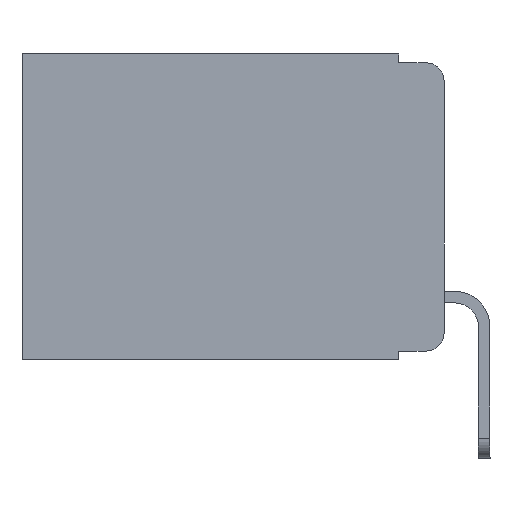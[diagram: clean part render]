
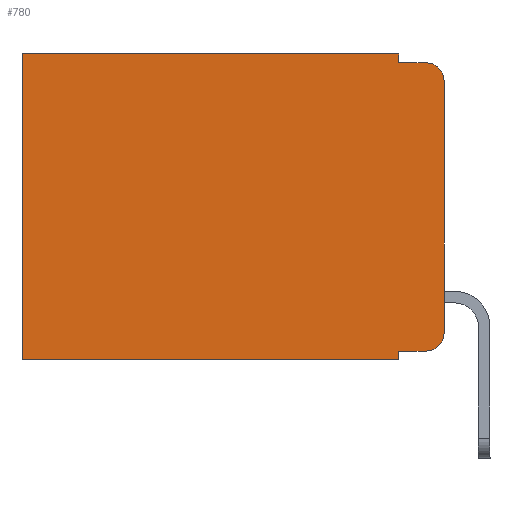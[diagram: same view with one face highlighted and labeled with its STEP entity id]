
A CAD part, left-side view. The second image highlights one B-rep face of the part: STEP entity #780.
In plain terms, the highlighted planar face has unit normal (-1, 0, 0).
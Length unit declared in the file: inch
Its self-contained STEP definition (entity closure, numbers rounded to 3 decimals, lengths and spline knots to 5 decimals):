
#149 = EDGE_CURVE ( 'NONE', #5123, #1282, #10667, .T. ) ;
#304 = EDGE_CURVE ( 'NONE', #12042, #5918, #4848, .T. ) ;
#460 = DIRECTION ( 'NONE',  ( 0., -1., 0. ) ) ;
#780 = ADVANCED_FACE ( 'NONE', ( #3816 ), #7426, .F. ) ;
#827 = CARTESIAN_POINT ( 'NONE',  ( 0.298, 0., -0.343 ) ) ;
#1242 = CARTESIAN_POINT ( 'NONE',  ( 0.298, 0.02, -0.03 ) ) ;
#1282 = VERTEX_POINT ( 'NONE', #5396 ) ;
#1289 = DIRECTION ( 'NONE',  ( 0., 0., -1. ) ) ;
#1403 = CARTESIAN_POINT ( 'NONE',  ( 0.298, 0.051, -0.01 ) ) ;
#1415 = CIRCLE ( 'NONE', #5154, 0.02 ) ;
#1849 = DIRECTION ( 'NONE',  ( 0., 1., 0. ) ) ;
#2070 = EDGE_CURVE ( 'NONE', #13044, #11261, #13061, .T. ) ;
#2125 = CARTESIAN_POINT ( 'NONE',  ( 0.298, 0.051, -0.333 ) ) ;
#2136 = VECTOR ( 'NONE', #10372, 39.37008 ) ;
#2192 = DIRECTION ( 'NONE',  ( 1., 0., 0. ) ) ;
#2296 = VECTOR ( 'NONE', #3104, 39.37008 ) ;
#2339 = CARTESIAN_POINT ( 'NONE',  ( 0.298, 0.051, -0.01 ) ) ;
#2659 = VECTOR ( 'NONE', #7117, 39.37008 ) ;
#2788 = LINE ( 'NONE', #7250, #11934 ) ;
#2936 = LINE ( 'NONE', #6293, #2296 ) ;
#2959 = VERTEX_POINT ( 'NONE', #5642 ) ;
#3104 = DIRECTION ( 'NONE',  ( 0., 0., -1. ) ) ;
#3174 = DIRECTION ( 'NONE',  ( 0., 0., -1. ) ) ;
#3342 = EDGE_CURVE ( 'NONE', #8020, #11632, #2936, .T. ) ;
#3527 = DIRECTION ( 'NONE',  ( 0., 0., -1. ) ) ;
#3816 = FACE_OUTER_BOUND ( 'NONE', #7843, .T. ) ;
#3938 = VECTOR ( 'NONE', #4885, 39.37008 ) ;
#4064 = ORIENTED_EDGE ( 'NONE', *, *, #5435, .T. ) ;
#4119 = AXIS2_PLACEMENT_3D ( 'NONE', #4359, #2192, #1289 ) ;
#4346 = EDGE_CURVE ( 'NONE', #5918, #2959, #9458, .T. ) ;
#4359 = CARTESIAN_POINT ( 'NONE',  ( 0.298, 0., 0. ) ) ;
#4547 = VERTEX_POINT ( 'NONE', #10240 ) ;
#4634 = CARTESIAN_POINT ( 'NONE',  ( 0.298, 0.051, 0. ) ) ;
#4745 = DIRECTION ( 'NONE',  ( -1., 0., 0. ) ) ;
#4821 = EDGE_CURVE ( 'NONE', #11632, #2959, #7723, .T. ) ;
#4848 = LINE ( 'NONE', #10439, #2136 ) ;
#4885 = DIRECTION ( 'NONE',  ( 0., -1., 0. ) ) ;
#4996 = VECTOR ( 'NONE', #3527, 39.37008 ) ;
#5123 = VERTEX_POINT ( 'NONE', #6391 ) ;
#5154 = AXIS2_PLACEMENT_3D ( 'NONE', #5719, #4745, #5676 ) ;
#5396 = CARTESIAN_POINT ( 'NONE',  ( 0.298, 0., -0.313 ) ) ;
#5435 = EDGE_CURVE ( 'NONE', #5123, #11261, #5818, .T. ) ;
#5642 = CARTESIAN_POINT ( 'NONE',  ( 0.298, 0.473, -0.343 ) ) ;
#5676 = DIRECTION ( 'NONE',  ( 0., 0., -1. ) ) ;
#5719 = CARTESIAN_POINT ( 'NONE',  ( 0.298, 0.02, -0.313 ) ) ;
#5786 = ORIENTED_EDGE ( 'NONE', *, *, #11718, .F. ) ;
#5818 = CIRCLE ( 'NONE', #8155, 0.02 ) ;
#5918 = VERTEX_POINT ( 'NONE', #10873 ) ;
#6119 = VECTOR ( 'NONE', #1849, 39.37008 ) ;
#6293 = CARTESIAN_POINT ( 'NONE',  ( 0.298, 0.051, 0. ) ) ;
#6391 = CARTESIAN_POINT ( 'NONE',  ( 0.298, 0., -0.03 ) ) ;
#6642 = CARTESIAN_POINT ( 'NONE',  ( 0.298, 0.051, -0.343 ) ) ;
#6697 = ORIENTED_EDGE ( 'NONE', *, *, #4821, .F. ) ;
#7117 = DIRECTION ( 'NONE',  ( 0., 0., -1. ) ) ;
#7190 = ORIENTED_EDGE ( 'NONE', *, *, #149, .F. ) ;
#7250 = CARTESIAN_POINT ( 'NONE',  ( 0.298, 0.051, 0. ) ) ;
#7426 = PLANE ( 'NONE',  #4119 ) ;
#7723 = LINE ( 'NONE', #827, #6119 ) ;
#7819 = ORIENTED_EDGE ( 'NONE', *, *, #9306, .T. ) ;
#7843 = EDGE_LOOP ( 'NONE', ( #7190, #4064, #8984, #5786, #9693, #8643, #6697, #10516, #7819, #8812 ) ) ;
#8020 = VERTEX_POINT ( 'NONE', #2125 ) ;
#8155 = AXIS2_PLACEMENT_3D ( 'NONE', #1242, #8303, #10005 ) ;
#8172 = CARTESIAN_POINT ( 'NONE',  ( 0.298, 0.473, 0. ) ) ;
#8303 = DIRECTION ( 'NONE',  ( -1., 0., 0. ) ) ;
#8528 = VECTOR ( 'NONE', #460, 39.37008 ) ;
#8643 = ORIENTED_EDGE ( 'NONE', *, *, #4346, .T. ) ;
#8812 = ORIENTED_EDGE ( 'NONE', *, *, #9688, .T. ) ;
#8984 = ORIENTED_EDGE ( 'NONE', *, *, #2070, .F. ) ;
#9306 = EDGE_CURVE ( 'NONE', #8020, #4547, #11655, .T. ) ;
#9458 = LINE ( 'NONE', #8172, #2659 ) ;
#9574 = CARTESIAN_POINT ( 'NONE',  ( 0.298, 0., 0. ) ) ;
#9688 = EDGE_CURVE ( 'NONE', #4547, #1282, #1415, .T. ) ;
#9693 = ORIENTED_EDGE ( 'NONE', *, *, #304, .T. ) ;
#10005 = DIRECTION ( 'NONE',  ( 0., 0., -1. ) ) ;
#10240 = CARTESIAN_POINT ( 'NONE',  ( 0.298, 0.02, -0.333 ) ) ;
#10372 = DIRECTION ( 'NONE',  ( 0., 1., 0. ) ) ;
#10439 = CARTESIAN_POINT ( 'NONE',  ( 0.298, 0., 0. ) ) ;
#10516 = ORIENTED_EDGE ( 'NONE', *, *, #3342, .F. ) ;
#10667 = LINE ( 'NONE', #9574, #4996 ) ;
#10873 = CARTESIAN_POINT ( 'NONE',  ( 0.298, 0.473, 0. ) ) ;
#11261 = VERTEX_POINT ( 'NONE', #12311 ) ;
#11632 = VERTEX_POINT ( 'NONE', #6642 ) ;
#11655 = LINE ( 'NONE', #11957, #3938 ) ;
#11718 = EDGE_CURVE ( 'NONE', #12042, #13044, #2788, .T. ) ;
#11934 = VECTOR ( 'NONE', #3174, 39.37008 ) ;
#11957 = CARTESIAN_POINT ( 'NONE',  ( 0.298, 0.051, -0.333 ) ) ;
#12042 = VERTEX_POINT ( 'NONE', #4634 ) ;
#12311 = CARTESIAN_POINT ( 'NONE',  ( 0.298, 0.02, -0.01 ) ) ;
#13044 = VERTEX_POINT ( 'NONE', #2339 ) ;
#13061 = LINE ( 'NONE', #1403, #8528 ) ;
